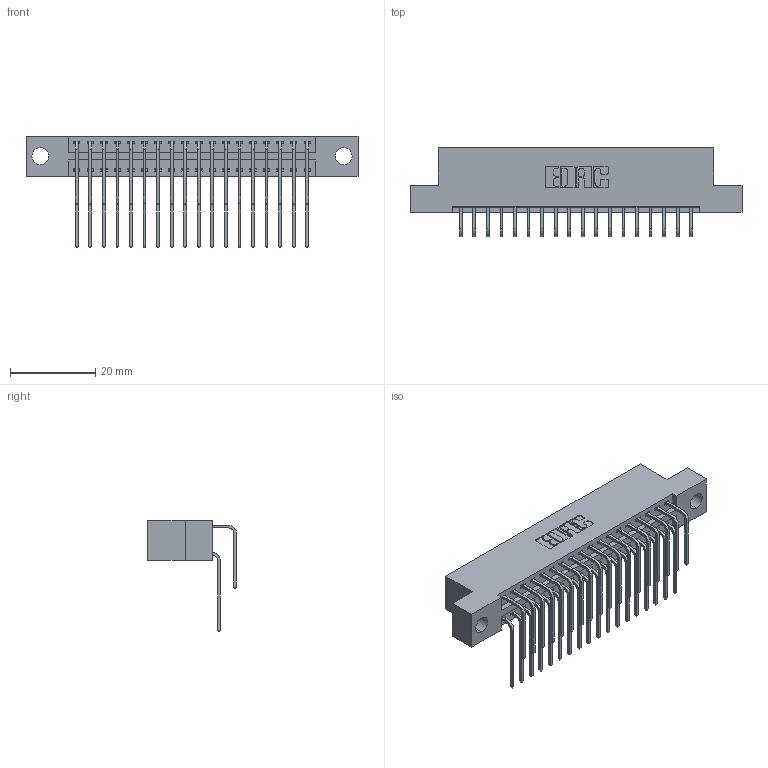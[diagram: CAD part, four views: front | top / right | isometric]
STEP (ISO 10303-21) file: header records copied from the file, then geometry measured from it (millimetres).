
FILE_DESCRIPTION (( 'STEP AP203' ), '1' );
FILE_NAME ('346-036-559-204.STEP', '2022-05-19T22:27:03', ( '' ), ( '' ), 'SwSTEP 2.0', 'SolidWorks 2020', '' );
FILE_SCHEMA (( 'CONFIG_CONTROL_DESIGN' ));
Length unit declared in the file: inch
Products named in the file (4): 346-036-559-204; 345-292-001_559 Tail - 2; 345-292-001_558 559 Tail - 1; 346 Part_Flush Mounting Lugs - 0.156 Dia-TH
Assembly tree (37 placements, depth 2):
  346-036-559-204
    346 Part_Flush Mounting Lugs - 0.156 Dia-TH
    345-292-001_558 559 Tail - 1  x18
    345-292-001_559 Tail - 2  x18
Bounding box: 77.72 x 20.89 x 26.16 mm (x, y, z)
Volume: 7494.4 mm3; surface area: 10768.5 mm2
Topology: 37 solids, 37 shells, 2080 faces, 6161 edges, 4058 vertices
Faces by surface type: plane 1422, cylinder 658
Entity records: 17181 total; most frequent: CARTESIAN_POINT 2921, ORIENTED_EDGE 2802, DIRECTION 2597, EDGE_CURVE 1401, VECTOR 1157, LINE 1157, VERTEX_POINT 930, AXIS2_PLACEMENT_3D 720
